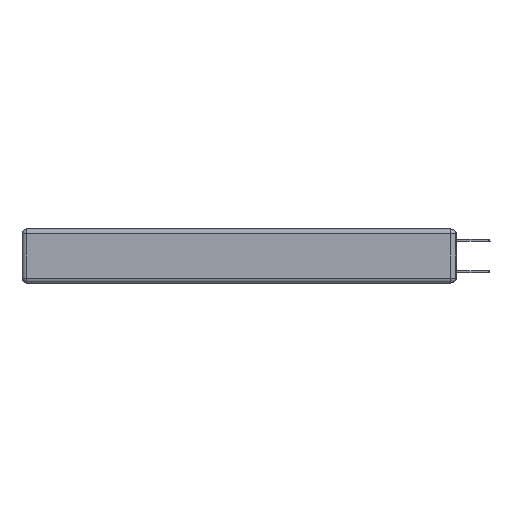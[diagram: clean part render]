
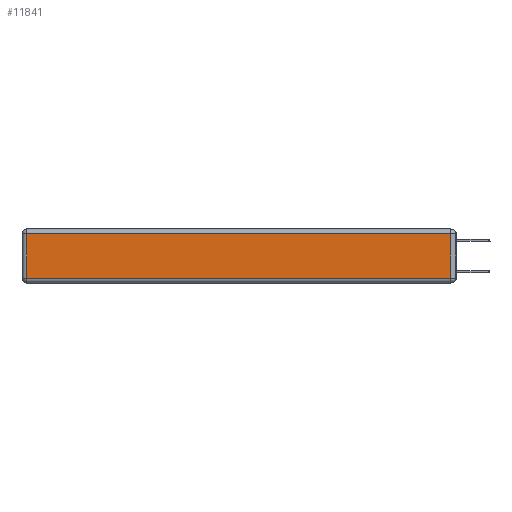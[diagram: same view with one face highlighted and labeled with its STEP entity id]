
A CAD part, left-side view. The second image highlights one B-rep face of the part: STEP entity #11841.
In plain terms, the highlighted planar face has unit normal (-1, 0, 0).
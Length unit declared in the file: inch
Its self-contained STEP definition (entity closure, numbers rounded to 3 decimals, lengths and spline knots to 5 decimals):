
#2002 = LINE ( 'NONE', #15186, #12284 ) ;
#2416 = PLANE ( 'NONE',  #7686 ) ;
#3200 = DIRECTION ( 'NONE',  ( 0., 0., -1. ) ) ;
#3211 = CARTESIAN_POINT ( 'NONE',  ( 0., 2.72, -0.03 ) ) ;
#3833 = DIRECTION ( 'NONE',  ( 0., 0., 1. ) ) ;
#4875 = EDGE_CURVE ( 'NONE', #11832, #5390, #2002, .T. ) ;
#5390 = VERTEX_POINT ( 'NONE', #3211 ) ;
#5588 = DIRECTION ( 'NONE',  ( 0., -1., 0. ) ) ;
#7140 = CARTESIAN_POINT ( 'NONE',  ( 0., 2.72, -0.313 ) ) ;
#7253 = LINE ( 'NONE', #8683, #7689 ) ;
#7686 = AXIS2_PLACEMENT_3D ( 'NONE', #16748, #16647, #3833 ) ;
#7689 = VECTOR ( 'NONE', #3200, 39.37008 ) ;
#7880 = FACE_OUTER_BOUND ( 'NONE', #15497, .T. ) ;
#8175 = VERTEX_POINT ( 'NONE', #17413 ) ;
#8542 = EDGE_CURVE ( 'NONE', #8175, #11832, #11355, .T. ) ;
#8683 = CARTESIAN_POINT ( 'NONE',  ( 0., 2.72, -0.343 ) ) ;
#9201 = VECTOR ( 'NONE', #5588, 39.37008 ) ;
#9458 = VECTOR ( 'NONE', #9748, 39.37008 ) ;
#9748 = DIRECTION ( 'NONE',  ( 0., 0., 1. ) ) ;
#9800 = EDGE_CURVE ( 'NONE', #11588, #8175, #18514, .T. ) ;
#10199 = ORIENTED_EDGE ( 'NONE', *, *, #8542, .T. ) ;
#10390 = EDGE_CURVE ( 'NONE', #5390, #11588, #7253, .T. ) ;
#11355 = LINE ( 'NONE', #14186, #9458 ) ;
#11375 = ORIENTED_EDGE ( 'NONE', *, *, #4875, .T. ) ;
#11534 = ORIENTED_EDGE ( 'NONE', *, *, #10390, .T. ) ;
#11588 = VERTEX_POINT ( 'NONE', #7140 ) ;
#11832 = VERTEX_POINT ( 'NONE', #12435 ) ;
#11841 = ADVANCED_FACE ( 'NONE', ( #7880 ), #2416, .T. ) ;
#12284 = VECTOR ( 'NONE', #13530, 39.37008 ) ;
#12337 = CARTESIAN_POINT ( 'NONE',  ( 0., 0., -0.313 ) ) ;
#12435 = CARTESIAN_POINT ( 'NONE',  ( 0., 0.03, -0.03 ) ) ;
#13530 = DIRECTION ( 'NONE',  ( 0., 1., 0. ) ) ;
#14186 = CARTESIAN_POINT ( 'NONE',  ( 0., 0.03, -0.343 ) ) ;
#14385 = ORIENTED_EDGE ( 'NONE', *, *, #9800, .T. ) ;
#15186 = CARTESIAN_POINT ( 'NONE',  ( 0., 2.75, -0.03 ) ) ;
#15497 = EDGE_LOOP ( 'NONE', ( #14385, #10199, #11375, #11534 ) ) ;
#16647 = DIRECTION ( 'NONE',  ( -1., 0., 0. ) ) ;
#16748 = CARTESIAN_POINT ( 'NONE',  ( 0., 0., -0.343 ) ) ;
#17413 = CARTESIAN_POINT ( 'NONE',  ( 0., 0.03, -0.313 ) ) ;
#18514 = LINE ( 'NONE', #12337, #9201 ) ;
